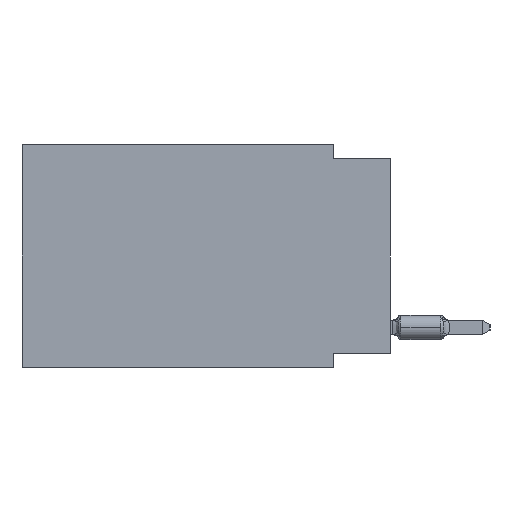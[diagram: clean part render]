
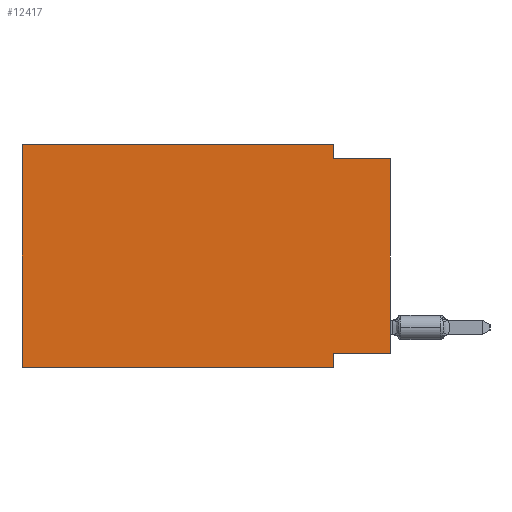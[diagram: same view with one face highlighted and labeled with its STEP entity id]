
A CAD part, left-side view. The second image highlights one B-rep face of the part: STEP entity #12417.
In plain terms, the highlighted planar face has unit normal (-1, 0, 0).
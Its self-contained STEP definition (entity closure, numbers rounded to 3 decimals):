
#2515 = VERTEX_POINT ( 'NONE', #30047 ) ;
#2742 = EDGE_CURVE ( 'NONE', #2515, #33251, #22714, .T. ) ;
#2898 = CARTESIAN_POINT ( 'NONE',  ( 0., 16.383, 0. ) ) ;
#6432 = EDGE_CURVE ( 'NONE', #24148, #60853, #22706, .T. ) ;
#9458 = DIRECTION ( 'NONE',  ( 0., -1., 0. ) ) ;
#10404 = DIRECTION ( 'NONE',  ( 0., 0., 1. ) ) ;
#10562 = VECTOR ( 'NONE', #37349, 1000. ) ;
#10668 = DIRECTION ( 'NONE',  ( 0., -1., 0. ) ) ;
#12417 = ADVANCED_FACE ( 'NONE', ( #19218 ), #14137, .F. ) ;
#14137 = PLANE ( 'NONE',  #14695 ) ;
#14199 = CARTESIAN_POINT ( 'NONE',  ( 0., 2.54, 0. ) ) ;
#14216 = CARTESIAN_POINT ( 'NONE',  ( 0., 2.54, 0. ) ) ;
#14695 = AXIS2_PLACEMENT_3D ( 'NONE', #2898, #23585, #18860 ) ;
#14938 = CARTESIAN_POINT ( 'NONE',  ( 0., 2.54, -9.906 ) ) ;
#15473 = VECTOR ( 'NONE', #26626, 1000. ) ;
#16081 = CARTESIAN_POINT ( 'NONE',  ( 0., 2.54, -0.635 ) ) ;
#16373 = ORIENTED_EDGE ( 'NONE', *, *, #24861, .F. ) ;
#16410 = VERTEX_POINT ( 'NONE', #16081 ) ;
#17740 = VECTOR ( 'NONE', #55029, 1000. ) ;
#18558 = VECTOR ( 'NONE', #10668, 1000. ) ;
#18860 = DIRECTION ( 'NONE',  ( 0., 0., -1. ) ) ;
#19218 = FACE_OUTER_BOUND ( 'NONE', #32969, .T. ) ;
#20332 = LINE ( 'NONE', #64509, #30876 ) ;
#20659 = CARTESIAN_POINT ( 'NONE',  ( 0., 2.54, -9.906 ) ) ;
#22706 = LINE ( 'NONE', #60027, #32357 ) ;
#22714 = LINE ( 'NONE', #33592, #44497 ) ;
#23585 = DIRECTION ( 'NONE',  ( 1., 0., 0. ) ) ;
#23967 = ORIENTED_EDGE ( 'NONE', *, *, #53059, .F. ) ;
#24148 = VERTEX_POINT ( 'NONE', #53748 ) ;
#24861 = EDGE_CURVE ( 'NONE', #16410, #60853, #66079, .T. ) ;
#26626 = DIRECTION ( 'NONE',  ( 0., 1., 0. ) ) ;
#26976 = LINE ( 'NONE', #54135, #15473 ) ;
#30047 = CARTESIAN_POINT ( 'NONE',  ( 0., 16.383, -9.906 ) ) ;
#30876 = VECTOR ( 'NONE', #9458, 1000. ) ;
#32357 = VECTOR ( 'NONE', #10404, 1000. ) ;
#32398 = ORIENTED_EDGE ( 'NONE', *, *, #41616, .F. ) ;
#32969 = EDGE_LOOP ( 'NONE', ( #36741, #16373, #23967, #60017, #48213, #48475, #49609, #32398 ) ) ;
#33251 = VERTEX_POINT ( 'NONE', #14938 ) ;
#33592 = CARTESIAN_POINT ( 'NONE',  ( 0., 16.383, -9.906 ) ) ;
#36741 = ORIENTED_EDGE ( 'NONE', *, *, #6432, .T. ) ;
#37349 = DIRECTION ( 'NONE',  ( 0., 0., -1. ) ) ;
#41616 = EDGE_CURVE ( 'NONE', #24148, #55306, #26976, .T. ) ;
#44167 = LINE ( 'NONE', #20659, #17740 ) ;
#44437 = DIRECTION ( 'NONE',  ( 0., -1., 0. ) ) ;
#44497 = VECTOR ( 'NONE', #44437, 1000. ) ;
#48213 = ORIENTED_EDGE ( 'NONE', *, *, #69399, .F. ) ;
#48475 = ORIENTED_EDGE ( 'NONE', *, *, #2742, .T. ) ;
#49609 = ORIENTED_EDGE ( 'NONE', *, *, #55410, .F. ) ;
#50655 = VERTEX_POINT ( 'NONE', #14216 ) ;
#53059 = EDGE_CURVE ( 'NONE', #50655, #16410, #63822, .T. ) ;
#53748 = CARTESIAN_POINT ( 'NONE',  ( 0., 0., -9.271 ) ) ;
#54135 = CARTESIAN_POINT ( 'NONE',  ( 0., 0., -9.271 ) ) ;
#54397 = CARTESIAN_POINT ( 'NONE',  ( 0., 16.383, 0. ) ) ;
#54409 = CARTESIAN_POINT ( 'NONE',  ( 0., 0., -0.635 ) ) ;
#55029 = DIRECTION ( 'NONE',  ( 0., 0., -1. ) ) ;
#55306 = VERTEX_POINT ( 'NONE', #69724 ) ;
#55410 = EDGE_CURVE ( 'NONE', #55306, #33251, #44167, .T. ) ;
#57621 = DIRECTION ( 'NONE',  ( 0., 0., 1. ) ) ;
#59601 = VERTEX_POINT ( 'NONE', #54397 ) ;
#60017 = ORIENTED_EDGE ( 'NONE', *, *, #64253, .F. ) ;
#60027 = CARTESIAN_POINT ( 'NONE',  ( 0., 0., 0. ) ) ;
#60166 = VECTOR ( 'NONE', #57621, 1000. ) ;
#60287 = CARTESIAN_POINT ( 'NONE',  ( 0., 0., -0.635 ) ) ;
#60853 = VERTEX_POINT ( 'NONE', #54409 ) ;
#63399 = LINE ( 'NONE', #67801, #60166 ) ;
#63822 = LINE ( 'NONE', #14199, #10562 ) ;
#64253 = EDGE_CURVE ( 'NONE', #59601, #50655, #20332, .T. ) ;
#64509 = CARTESIAN_POINT ( 'NONE',  ( 0., 16.383, 0. ) ) ;
#66079 = LINE ( 'NONE', #60287, #18558 ) ;
#67801 = CARTESIAN_POINT ( 'NONE',  ( 0., 16.383, 0. ) ) ;
#69399 = EDGE_CURVE ( 'NONE', #2515, #59601, #63399, .T. ) ;
#69724 = CARTESIAN_POINT ( 'NONE',  ( 0., 2.54, -9.271 ) ) ;
